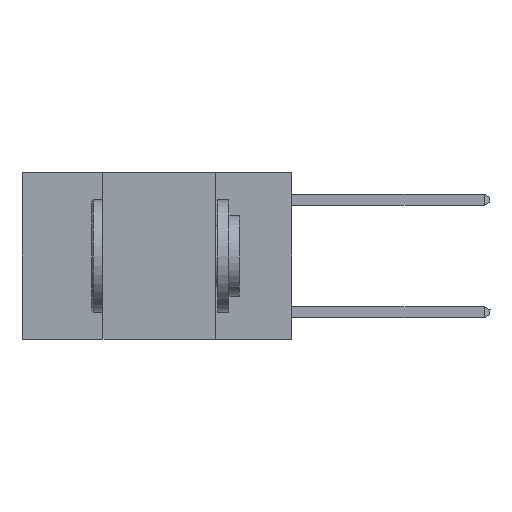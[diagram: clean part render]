
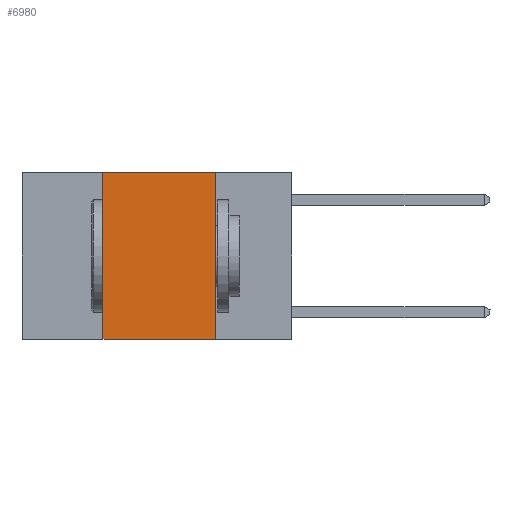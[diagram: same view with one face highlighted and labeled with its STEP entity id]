
A CAD part, left-side view. The second image highlights one B-rep face of the part: STEP entity #6980.
In plain terms, the highlighted planar face has unit normal (-1, 0, 0).
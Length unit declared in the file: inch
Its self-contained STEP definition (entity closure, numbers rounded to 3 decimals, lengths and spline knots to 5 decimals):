
#148 = DIRECTION ( 'NONE',  ( 0., 0., 1. ) ) ;
#344 = VERTEX_POINT ( 'NONE', #16310 ) ;
#895 = CARTESIAN_POINT ( 'NONE',  ( 0., 0.17, 0. ) ) ;
#2118 = LINE ( 'NONE', #11235, #10217 ) ;
#2736 = EDGE_LOOP ( 'NONE', ( #10632, #19072, #15286, #8386 ) ) ;
#4226 = CARTESIAN_POINT ( 'NONE',  ( 0., 0.17, 0. ) ) ;
#4797 = CARTESIAN_POINT ( 'NONE',  ( 0., 0.6, -0.37 ) ) ;
#4917 = DIRECTION ( 'NONE',  ( 0., -1., 0. ) ) ;
#5653 = EDGE_CURVE ( 'NONE', #6616, #12122, #11779, .T. ) ;
#5871 = DIRECTION ( 'NONE',  ( 0., 0., -1. ) ) ;
#5929 = DIRECTION ( 'NONE',  ( 0., 0., -1. ) ) ;
#6110 = CARTESIAN_POINT ( 'NONE',  ( 0., 0.42, -0.37 ) ) ;
#6449 = DIRECTION ( 'NONE',  ( 0., -1., 0. ) ) ;
#6616 = VERTEX_POINT ( 'NONE', #18400 ) ;
#6980 = ADVANCED_FACE ( 'NONE', ( #8466 ), #12143, .F. ) ;
#7990 = VECTOR ( 'NONE', #5871, 39.37008 ) ;
#8386 = ORIENTED_EDGE ( 'NONE', *, *, #15006, .T. ) ;
#8466 = FACE_OUTER_BOUND ( 'NONE', #2736, .T. ) ;
#10217 = VECTOR ( 'NONE', #148, 39.37008 ) ;
#10414 = AXIS2_PLACEMENT_3D ( 'NONE', #18131, #15103, #5929 ) ;
#10536 = LINE ( 'NONE', #4226, #7990 ) ;
#10632 = ORIENTED_EDGE ( 'NONE', *, *, #15358, .F. ) ;
#11235 = CARTESIAN_POINT ( 'NONE',  ( 0., 0.42, 0. ) ) ;
#11559 = LINE ( 'NONE', #4797, #14525 ) ;
#11779 = LINE ( 'NONE', #18760, #19721 ) ;
#12122 = VERTEX_POINT ( 'NONE', #895 ) ;
#12143 = PLANE ( 'NONE',  #10414 ) ;
#14525 = VECTOR ( 'NONE', #6449, 39.37008 ) ;
#15006 = EDGE_CURVE ( 'NONE', #16734, #344, #11559, .T. ) ;
#15033 = EDGE_CURVE ( 'NONE', #16734, #6616, #2118, .T. ) ;
#15103 = DIRECTION ( 'NONE',  ( 1., 0., 0. ) ) ;
#15286 = ORIENTED_EDGE ( 'NONE', *, *, #15033, .F. ) ;
#15358 = EDGE_CURVE ( 'NONE', #12122, #344, #10536, .T. ) ;
#16310 = CARTESIAN_POINT ( 'NONE',  ( 0., 0.17, -0.37 ) ) ;
#16734 = VERTEX_POINT ( 'NONE', #6110 ) ;
#18131 = CARTESIAN_POINT ( 'NONE',  ( 0., 0.6, 0. ) ) ;
#18400 = CARTESIAN_POINT ( 'NONE',  ( 0., 0.42, 0. ) ) ;
#18760 = CARTESIAN_POINT ( 'NONE',  ( 0., 0.6, 0. ) ) ;
#19072 = ORIENTED_EDGE ( 'NONE', *, *, #5653, .F. ) ;
#19721 = VECTOR ( 'NONE', #4917, 39.37008 ) ;
